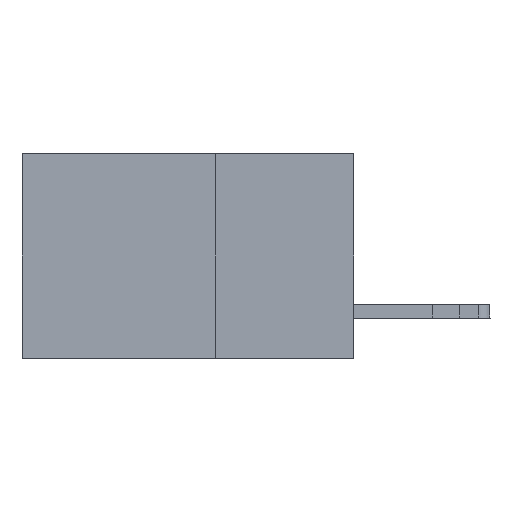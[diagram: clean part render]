
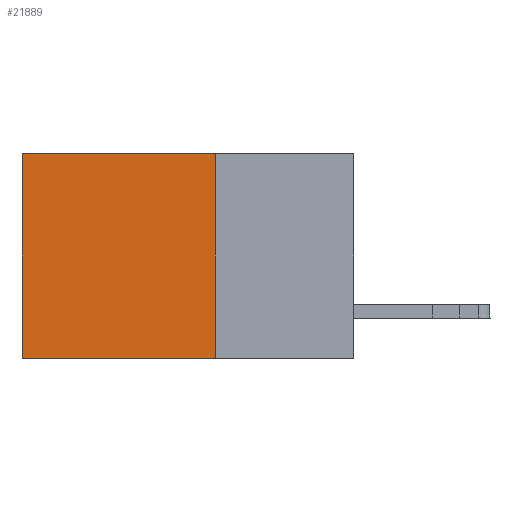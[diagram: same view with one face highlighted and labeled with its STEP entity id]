
A CAD part, left-side view. The second image highlights one B-rep face of the part: STEP entity #21889.
In plain terms, the highlighted planar face has unit normal (-1, 0, 0).
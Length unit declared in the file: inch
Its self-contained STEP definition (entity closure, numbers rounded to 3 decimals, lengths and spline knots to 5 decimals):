
#565 = CARTESIAN_POINT ( 'NONE',  ( 0.2875, 0.6, 0. ) ) ;
#2053 = EDGE_CURVE ( 'NONE', #4804, #5670, #38849, .T. ) ;
#4362 = ORIENTED_EDGE ( 'NONE', *, *, #37976, .T. ) ;
#4804 = VERTEX_POINT ( 'NONE', #31660 ) ;
#4988 = LINE ( 'NONE', #20562, #27018 ) ;
#5670 = VERTEX_POINT ( 'NONE', #23099 ) ;
#6873 = ORIENTED_EDGE ( 'NONE', *, *, #2053, .F. ) ;
#8252 = ORIENTED_EDGE ( 'NONE', *, *, #8278, .F. ) ;
#8278 = EDGE_CURVE ( 'NONE', #29039, #4804, #36888, .T. ) ;
#8603 = LINE ( 'NONE', #17566, #32895 ) ;
#10686 = CARTESIAN_POINT ( 'NONE',  ( 0.2875, 0.25, 0. ) ) ;
#13079 = DIRECTION ( 'NONE',  ( 0., 0., -1. ) ) ;
#13668 = VERTEX_POINT ( 'NONE', #565 ) ;
#14294 = PLANE ( 'NONE',  #36508 ) ;
#17103 = FACE_OUTER_BOUND ( 'NONE', #37297, .T. ) ;
#17441 = CARTESIAN_POINT ( 'NONE',  ( 0.2875, 0.25, -0.37 ) ) ;
#17566 = CARTESIAN_POINT ( 'NONE',  ( 0.2875, 0.6, 0. ) ) ;
#20562 = CARTESIAN_POINT ( 'NONE',  ( 0.2875, 0.25, 0. ) ) ;
#20772 = DIRECTION ( 'NONE',  ( 0., 0., -1. ) ) ;
#21721 = VECTOR ( 'NONE', #29834, 39.37008 ) ;
#21889 = ADVANCED_FACE ( 'NONE', ( #17103 ), #14294, .F. ) ;
#23099 = CARTESIAN_POINT ( 'NONE',  ( 0.2875, 0.6, -0.37 ) ) ;
#23108 = CARTESIAN_POINT ( 'NONE',  ( 0.2875, 0.25, 0. ) ) ;
#27018 = VECTOR ( 'NONE', #29158, 39.37008 ) ;
#29039 = VERTEX_POINT ( 'NONE', #10686 ) ;
#29158 = DIRECTION ( 'NONE',  ( 0., 1., 0. ) ) ;
#29292 = DIRECTION ( 'NONE',  ( 1., 0., 0. ) ) ;
#29529 = ORIENTED_EDGE ( 'NONE', *, *, #36753, .T. ) ;
#29834 = DIRECTION ( 'NONE',  ( 0., 1., 0. ) ) ;
#31660 = CARTESIAN_POINT ( 'NONE',  ( 0.2875, 0.25, -0.37 ) ) ;
#31842 = VECTOR ( 'NONE', #13079, 39.37008 ) ;
#32895 = VECTOR ( 'NONE', #20772, 39.37008 ) ;
#36508 = AXIS2_PLACEMENT_3D ( 'NONE', #23108, #29292, #38687 ) ;
#36753 = EDGE_CURVE ( 'NONE', #29039, #13668, #4988, .T. ) ;
#36888 = LINE ( 'NONE', #37868, #31842 ) ;
#37297 = EDGE_LOOP ( 'NONE', ( #4362, #6873, #8252, #29529 ) ) ;
#37868 = CARTESIAN_POINT ( 'NONE',  ( 0.2875, 0.25, 0. ) ) ;
#37976 = EDGE_CURVE ( 'NONE', #13668, #5670, #8603, .T. ) ;
#38687 = DIRECTION ( 'NONE',  ( 0., 0., -1. ) ) ;
#38849 = LINE ( 'NONE', #17441, #21721 ) ;
